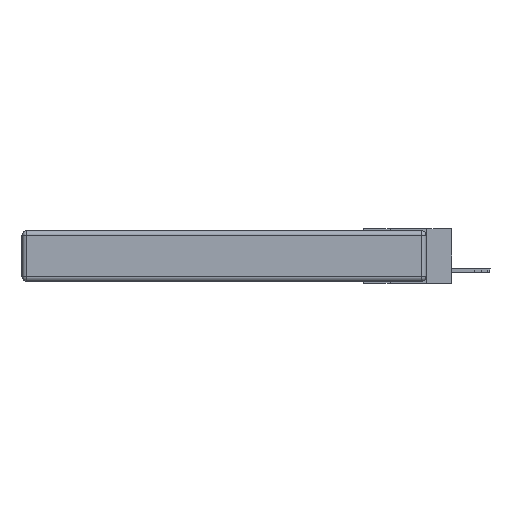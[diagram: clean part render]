
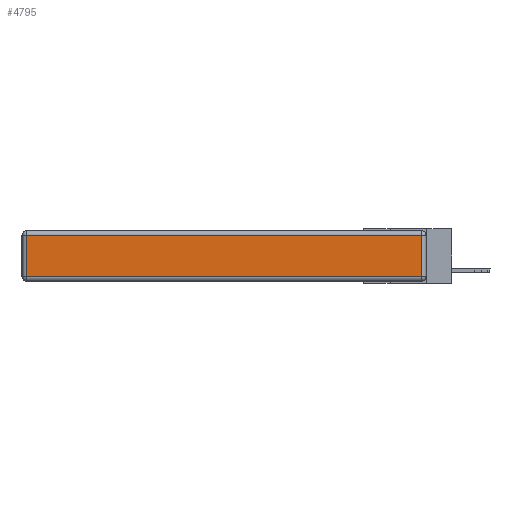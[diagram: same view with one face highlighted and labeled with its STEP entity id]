
A CAD part, left-side view. The second image highlights one B-rep face of the part: STEP entity #4795.
In plain terms, the highlighted planar face has unit normal (-1, 0, 0).
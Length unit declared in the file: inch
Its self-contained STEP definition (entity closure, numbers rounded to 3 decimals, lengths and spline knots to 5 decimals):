
#344 = DIRECTION ( 'NONE',  ( 0., -1., 0. ) ) ;
#1351 = VECTOR ( 'NONE', #1927, 39.37008 ) ;
#1380 = CARTESIAN_POINT ( 'NONE',  ( 0., 0.03, -0.343 ) ) ;
#1542 = VERTEX_POINT ( 'NONE', #16466 ) ;
#1686 = CARTESIAN_POINT ( 'NONE',  ( 0., 2.72, -0.03 ) ) ;
#1927 = DIRECTION ( 'NONE',  ( 0., 0., -1. ) ) ;
#3208 = CARTESIAN_POINT ( 'NONE',  ( 0., 2.75, -0.03 ) ) ;
#4795 = ADVANCED_FACE ( 'NONE', ( #11527 ), #5145, .T. ) ;
#5145 = PLANE ( 'NONE',  #10907 ) ;
#5844 = VERTEX_POINT ( 'NONE', #1686 ) ;
#6683 = EDGE_CURVE ( 'NONE', #1542, #5844, #22261, .T. ) ;
#6938 = ORIENTED_EDGE ( 'NONE', *, *, #20457, .T. ) ;
#7125 = VECTOR ( 'NONE', #9986, 39.37008 ) ;
#7359 = VECTOR ( 'NONE', #13295, 39.37008 ) ;
#8865 = CARTESIAN_POINT ( 'NONE',  ( 0., 0., -0.313 ) ) ;
#9513 = CARTESIAN_POINT ( 'NONE',  ( 0., 2.72, -0.343 ) ) ;
#9986 = DIRECTION ( 'NONE',  ( 0., 1., 0. ) ) ;
#10188 = ORIENTED_EDGE ( 'NONE', *, *, #6683, .T. ) ;
#10869 = CARTESIAN_POINT ( 'NONE',  ( 0., 2.72, -0.313 ) ) ;
#10907 = AXIS2_PLACEMENT_3D ( 'NONE', #11944, #20613, #22221 ) ;
#11366 = ORIENTED_EDGE ( 'NONE', *, *, #20836, .T. ) ;
#11407 = LINE ( 'NONE', #1380, #7359 ) ;
#11527 = FACE_OUTER_BOUND ( 'NONE', #22153, .T. ) ;
#11679 = LINE ( 'NONE', #8865, #16818 ) ;
#11944 = CARTESIAN_POINT ( 'NONE',  ( 0., 0., -0.343 ) ) ;
#13295 = DIRECTION ( 'NONE',  ( 0., 0., 1. ) ) ;
#14861 = LINE ( 'NONE', #9513, #1351 ) ;
#16025 = VERTEX_POINT ( 'NONE', #10869 ) ;
#16221 = ORIENTED_EDGE ( 'NONE', *, *, #16288, .T. ) ;
#16288 = EDGE_CURVE ( 'NONE', #5844, #16025, #14861, .T. ) ;
#16466 = CARTESIAN_POINT ( 'NONE',  ( 0., 0.03, -0.03 ) ) ;
#16818 = VECTOR ( 'NONE', #344, 39.37008 ) ;
#19680 = CARTESIAN_POINT ( 'NONE',  ( 0., 0.03, -0.313 ) ) ;
#20457 = EDGE_CURVE ( 'NONE', #16025, #21295, #11679, .T. ) ;
#20613 = DIRECTION ( 'NONE',  ( -1., 0., 0. ) ) ;
#20836 = EDGE_CURVE ( 'NONE', #21295, #1542, #11407, .T. ) ;
#21295 = VERTEX_POINT ( 'NONE', #19680 ) ;
#22153 = EDGE_LOOP ( 'NONE', ( #6938, #11366, #10188, #16221 ) ) ;
#22221 = DIRECTION ( 'NONE',  ( 0., 0., 1. ) ) ;
#22261 = LINE ( 'NONE', #3208, #7125 ) ;
